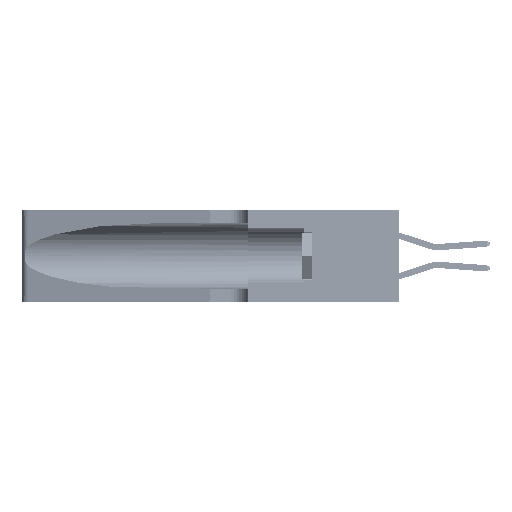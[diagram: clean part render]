
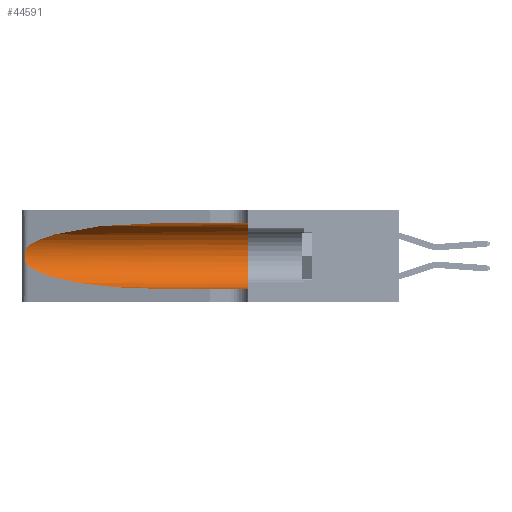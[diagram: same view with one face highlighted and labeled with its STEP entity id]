
A CAD part, left-side view. The second image highlights one B-rep face of the part: STEP entity #44591.
In plain terms, the highlighted cylindrical face has radius 3.308 mm (diameter 6.617 mm), a partial arc.
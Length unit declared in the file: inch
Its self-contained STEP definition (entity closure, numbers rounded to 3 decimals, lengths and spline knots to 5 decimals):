
#958 =( BOUNDED_CURVE ( )  B_SPLINE_CURVE ( 3, ( #26222, #47208, #34784, #9394 ),
 .UNSPECIFIED., .F., .F. ) 
 B_SPLINE_CURVE_WITH_KNOTS ( ( 4, 4 ),
 ( 3.44316, 4.71239 ),
 .UNSPECIFIED. ) 
 CURVE ( )  GEOMETRIC_REPRESENTATION_ITEM ( )  RATIONAL_B_SPLINE_CURVE ( ( 1., 0.87, 0.87, 1. ) ) 
 REPRESENTATION_ITEM ( '' )  );
#1930 = DIRECTION ( 'NONE',  ( 0., 1., 0. ) ) ;
#1951 = CARTESIAN_POINT ( 'NONE',  ( 0.25487, 1.22718, 0.22369 ) ) ;
#2130 = CARTESIAN_POINT ( 'NONE',  ( 0.25854, 1.2359, 0.20912 ) ) ;
#2816 = DIRECTION ( 'NONE',  ( 0., -1., 0. ) ) ;
#4253 = CARTESIAN_POINT ( 'NONE',  ( 0.1305, 0.35, 0.31525 ) ) ;
#4477 = LINE ( 'NONE', #23483, #13194 ) ;
#4971 = AXIS2_PLACEMENT_3D ( 'NONE', #27434, #1930, #31729 ) ;
#5471 = EDGE_CURVE ( 'NONE', #24260, #22460, #21497, .T. ) ;
#6483 = CARTESIAN_POINT ( 'NONE',  ( 0.26075, 1.23896, 0.19203 ) ) ;
#6788 = ORIENTED_EDGE ( 'NONE', *, *, #20052, .F. ) ;
#6839 = CARTESIAN_POINT ( 'NONE',  ( 0.2373, 1.15595, 0.28018 ) ) ;
#7857 = CARTESIAN_POINT ( 'NONE',  ( 0.1305, 0.72297, 0.31525 ) ) ;
#8043 = CARTESIAN_POINT ( 'NONE',  ( 0.25487, 1.22718, 0.14631 ) ) ;
#9394 = CARTESIAN_POINT ( 'NONE',  ( 0.1305, 0.72297, 0.05475 ) ) ;
#9534 = VERTEX_POINT ( 'NONE', #8043 ) ;
#10817 = CARTESIAN_POINT ( 'NONE',  ( 0.26017, 1.23833, 0.17102 ) ) ;
#11477 = CARTESIAN_POINT ( 'NONE',  ( 0.1305, 1.61858, 0.185 ) ) ;
#13194 = VECTOR ( 'NONE', #27762, 39.37008 ) ;
#14121 = CARTESIAN_POINT ( 'NONE',  ( 0.25487, 1.22718, 0.22369 ) ) ;
#15061 = CARTESIAN_POINT ( 'NONE',  ( 0.25789, 1.23486, 0.15765 ) ) ;
#16758 = ORIENTED_EDGE ( 'NONE', *, *, #42678, .T. ) ;
#16770 =( BOUNDED_CURVE ( )  B_SPLINE_CURVE ( 3, ( #48893, #27970, #6839, #36508 ),
 .UNSPECIFIED., .F., .F. ) 
 B_SPLINE_CURVE_WITH_KNOTS ( ( 4, 4 ),
 ( 1.5708, 2.84003 ),
 .UNSPECIFIED. ) 
 CURVE ( )  GEOMETRIC_REPRESENTATION_ITEM ( )  RATIONAL_B_SPLINE_CURVE ( ( 1., 0.87, 0.87, 1. ) ) 
 REPRESENTATION_ITEM ( '' )  );
#17295 = VERTEX_POINT ( 'NONE', #36976 ) ;
#19287 = CARTESIAN_POINT ( 'NONE',  ( 0.25555, 1.22993, 0.14849 ) ) ;
#20052 = EDGE_CURVE ( 'NONE', #22460, #17295, #30771, .T. ) ;
#21079 = EDGE_CURVE ( 'NONE', #9534, #35129, #958, .T. ) ;
#21497 = LINE ( 'NONE', #34119, #53674 ) ;
#22460 = VERTEX_POINT ( 'NONE', #4253 ) ;
#23120 = AXIS2_PLACEMENT_3D ( 'NONE', #11477, #2816, #32606 ) ;
#23483 = CARTESIAN_POINT ( 'NONE',  ( 0.1305, 1.61858, 0.05475 ) ) ;
#24026 = ORIENTED_EDGE ( 'NONE', *, *, #46554, .T. ) ;
#24260 = VERTEX_POINT ( 'NONE', #7857 ) ;
#26222 = CARTESIAN_POINT ( 'NONE',  ( 0.25487, 1.22718, 0.14631 ) ) ;
#26681 = ORIENTED_EDGE ( 'NONE', *, *, #21079, .T. ) ;
#27434 = CARTESIAN_POINT ( 'NONE',  ( 0.1305, 0.35, 0.185 ) ) ;
#27637 = CARTESIAN_POINT ( 'NONE',  ( 0.25787, 1.23484, 0.2124 ) ) ;
#27762 = DIRECTION ( 'NONE',  ( 0., -1., 0. ) ) ;
#27970 = CARTESIAN_POINT ( 'NONE',  ( 0.18966, 0.96281, 0.31525 ) ) ;
#30771 = CIRCLE ( 'NONE', #4971, 0.13025 ) ;
#31729 = DIRECTION ( 'NONE',  ( 0., 0., 1. ) ) ;
#31929 = CARTESIAN_POINT ( 'NONE',  ( 0.26018, 1.23835, 0.19895 ) ) ;
#32606 = DIRECTION ( 'NONE',  ( 0., 0., -1. ) ) ;
#32879 = FACE_OUTER_BOUND ( 'NONE', #36865, .T. ) ;
#34012 = ORIENTED_EDGE ( 'NONE', *, *, #43966, .T. ) ;
#34119 = CARTESIAN_POINT ( 'NONE',  ( 0.1305, 1.61858, 0.31525 ) ) ;
#34784 = CARTESIAN_POINT ( 'NONE',  ( 0.18966, 0.96281, 0.05475 ) ) ;
#35129 = VERTEX_POINT ( 'NONE', #48638 ) ;
#36175 = CARTESIAN_POINT ( 'NONE',  ( 0.26075, 1.23896, 0.178 ) ) ;
#36508 = CARTESIAN_POINT ( 'NONE',  ( 0.25487, 1.22718, 0.22369 ) ) ;
#36865 = EDGE_LOOP ( 'NONE', ( #34012, #24026, #26681, #16758, #6788, #45813 ) ) ;
#36976 = CARTESIAN_POINT ( 'NONE',  ( 0.1305, 0.35, 0.05475 ) ) ;
#38288 = DIRECTION ( 'NONE',  ( 0., -1., 0. ) ) ;
#40059 = CYLINDRICAL_SURFACE ( 'NONE', #23120, 0.13025 ) ;
#40168 = CARTESIAN_POINT ( 'NONE',  ( 0.25555, 1.22994, 0.2215 ) ) ;
#40355 = CARTESIAN_POINT ( 'NONE',  ( 0.25856, 1.23593, 0.16098 ) ) ;
#42678 = EDGE_CURVE ( 'NONE', #35129, #17295, #4477, .T. ) ;
#43966 = EDGE_CURVE ( 'NONE', #24260, #53263, #16770, .T. ) ;
#44563 = CARTESIAN_POINT ( 'NONE',  ( 0.25639, 1.23186, 0.15144 ) ) ;
#44591 = ADVANCED_FACE ( 'NONE', ( #32879 ), #40059, .F. ) ;
#45813 = ORIENTED_EDGE ( 'NONE', *, *, #5471, .F. ) ;
#46554 = EDGE_CURVE ( 'NONE', #53263, #9534, #51797, .T. ) ;
#47208 = CARTESIAN_POINT ( 'NONE',  ( 0.2373, 1.15595, 0.08982 ) ) ;
#48638 = CARTESIAN_POINT ( 'NONE',  ( 0.1305, 0.72297, 0.05475 ) ) ;
#48742 = CARTESIAN_POINT ( 'NONE',  ( 0.25487, 1.22718, 0.14631 ) ) ;
#48893 = CARTESIAN_POINT ( 'NONE',  ( 0.1305, 0.72297, 0.31525 ) ) ;
#51797 = B_SPLINE_CURVE_WITH_KNOTS ( 'NONE', 3,
 ( #1951, #40168, #52714, #27637, #2130, #31929, #6483, #36175, #10817, #40355, #15061, #44563, #19287, #48742 ),
 .UNSPECIFIED., .F., .F.,
 ( 4, 2, 2, 2, 2, 2, 4 ),
 ( 0., 0.00027, 0.00053, 0.00107, 0.0016, 0.00187, 0.00214 ),
 .UNSPECIFIED. ) ;
#52714 = CARTESIAN_POINT ( 'NONE',  ( 0.25639, 1.23184, 0.21858 ) ) ;
#53263 = VERTEX_POINT ( 'NONE', #14121 ) ;
#53674 = VECTOR ( 'NONE', #38288, 39.37008 ) ;
